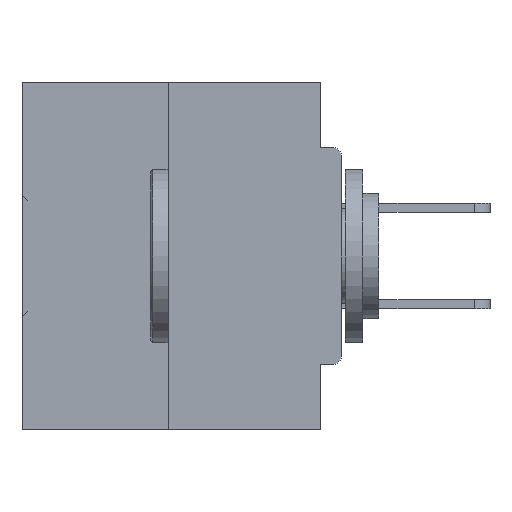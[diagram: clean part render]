
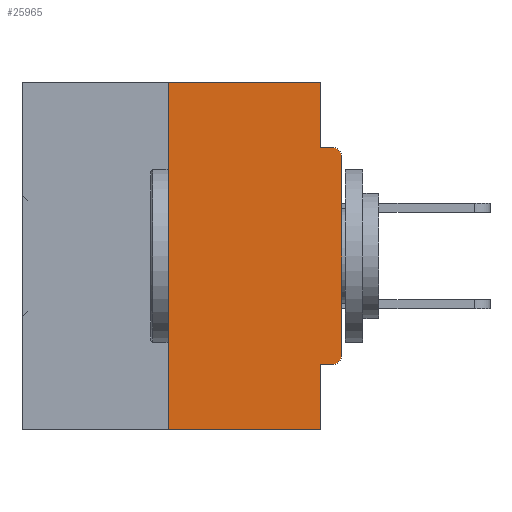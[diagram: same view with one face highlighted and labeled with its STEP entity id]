
A CAD part, left-side view. The second image highlights one B-rep face of the part: STEP entity #25965.
In plain terms, the highlighted planar face has unit normal (-1, 0, 0).
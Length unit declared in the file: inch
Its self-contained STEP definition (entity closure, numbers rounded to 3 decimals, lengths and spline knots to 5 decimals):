
#88 = VERTEX_POINT ( 'NONE', #2777 ) ;
#303 = EDGE_CURVE ( 'NONE', #88, #38447, #35368, .T. ) ;
#573 = CARTESIAN_POINT ( 'NONE',  ( 0., 0.015, -0.1085 ) ) ;
#939 = VERTEX_POINT ( 'NONE', #4171 ) ;
#961 = CARTESIAN_POINT ( 'NONE',  ( 0., 0., 0. ) ) ;
#1025 = VECTOR ( 'NONE', #41453, 39.37008 ) ;
#1994 = LINE ( 'NONE', #46334, #4847 ) ;
#2709 = ORIENTED_EDGE ( 'NONE', *, *, #18838, .T. ) ;
#2777 = CARTESIAN_POINT ( 'NONE',  ( 0., 0.015, -0.4065 ) ) ;
#3264 = LINE ( 'NONE', #10481, #41026 ) ;
#3377 = CARTESIAN_POINT ( 'NONE',  ( 0., 0.031, 0. ) ) ;
#3572 = CARTESIAN_POINT ( 'NONE',  ( 0., 0.031, -0.0935 ) ) ;
#4171 = CARTESIAN_POINT ( 'NONE',  ( 0., 0.031, 0. ) ) ;
#4847 = VECTOR ( 'NONE', #24423, 39.37008 ) ;
#6407 = ORIENTED_EDGE ( 'NONE', *, *, #303, .T. ) ;
#7286 = CARTESIAN_POINT ( 'NONE',  ( 0., 0., -0.0935 ) ) ;
#7782 = CARTESIAN_POINT ( 'NONE',  ( 0., 0.46, 0. ) ) ;
#8042 = DIRECTION ( 'NONE',  ( 0., 0., 1. ) ) ;
#8461 = CARTESIAN_POINT ( 'NONE',  ( 0., 0.031, -0.4065 ) ) ;
#8594 = VECTOR ( 'NONE', #8042, 39.37008 ) ;
#8871 = VECTOR ( 'NONE', #10265, 39.37008 ) ;
#9704 = DIRECTION ( 'NONE',  ( 0., -1., 0. ) ) ;
#10016 = AXIS2_PLACEMENT_3D ( 'NONE', #37822, #11801, #41209 ) ;
#10265 = DIRECTION ( 'NONE',  ( 0., 0., -1. ) ) ;
#10481 = CARTESIAN_POINT ( 'NONE',  ( 0., 0.031, -0.5 ) ) ;
#10542 = CARTESIAN_POINT ( 'NONE',  ( 0., 0., -0.1085 ) ) ;
#11445 = DIRECTION ( 'NONE',  ( 0., -1., 0. ) ) ;
#11801 = DIRECTION ( 'NONE',  ( 1., 0., 0. ) ) ;
#12093 = AXIS2_PLACEMENT_3D ( 'NONE', #573, #18956, #22210 ) ;
#12139 = CARTESIAN_POINT ( 'NONE',  ( 0., 0.25, 0. ) ) ;
#13243 = ORIENTED_EDGE ( 'NONE', *, *, #16351, .T. ) ;
#13870 = CARTESIAN_POINT ( 'NONE',  ( 0., 0.46, -0.5 ) ) ;
#14209 = LINE ( 'NONE', #7286, #1025 ) ;
#14239 = VERTEX_POINT ( 'NONE', #3572 ) ;
#15760 = ORIENTED_EDGE ( 'NONE', *, *, #34628, .F. ) ;
#15966 = VERTEX_POINT ( 'NONE', #8461 ) ;
#16351 = EDGE_CURVE ( 'NONE', #38447, #18301, #37714, .T. ) ;
#16870 = EDGE_CURVE ( 'NONE', #14239, #40685, #14209, .T. ) ;
#17230 = VECTOR ( 'NONE', #11445, 39.37008 ) ;
#18301 = VERTEX_POINT ( 'NONE', #10542 ) ;
#18449 = CARTESIAN_POINT ( 'NONE',  ( 0., 0.25, -0.5 ) ) ;
#18695 = FACE_OUTER_BOUND ( 'NONE', #36446, .T. ) ;
#18838 = EDGE_CURVE ( 'NONE', #18301, #40685, #26674, .T. ) ;
#18956 = DIRECTION ( 'NONE',  ( -1., 0., 0. ) ) ;
#19839 = EDGE_CURVE ( 'NONE', #88, #15966, #1994, .T. ) ;
#21056 = CARTESIAN_POINT ( 'NONE',  ( 0., 0., -0.3915 ) ) ;
#21159 = VECTOR ( 'NONE', #33905, 39.37008 ) ;
#22210 = DIRECTION ( 'NONE',  ( 0., 0., -1. ) ) ;
#22990 = EDGE_CURVE ( 'NONE', #35570, #28768, #33197, .T. ) ;
#23413 = ORIENTED_EDGE ( 'NONE', *, *, #46625, .F. ) ;
#24423 = DIRECTION ( 'NONE',  ( 0., 1., 0. ) ) ;
#25965 = ADVANCED_FACE ( 'NONE', ( #18695 ), #30326, .F. ) ;
#26558 = ORIENTED_EDGE ( 'NONE', *, *, #19839, .F. ) ;
#26566 = CARTESIAN_POINT ( 'NONE',  ( 0., 0.25, 0. ) ) ;
#26674 = CIRCLE ( 'NONE', #12093, 0.015 ) ;
#27785 = LINE ( 'NONE', #3377, #8871 ) ;
#28768 = VERTEX_POINT ( 'NONE', #12139 ) ;
#29153 = CARTESIAN_POINT ( 'NONE',  ( 0., 0.015, -0.0935 ) ) ;
#29648 = EDGE_CURVE ( 'NONE', #35570, #39472, #45876, .T. ) ;
#30326 = PLANE ( 'NONE',  #10016 ) ;
#30826 = DIRECTION ( 'NONE',  ( 0., 0., -1. ) ) ;
#31485 = CARTESIAN_POINT ( 'NONE',  ( 0., 0.015, -0.3915 ) ) ;
#31565 = LINE ( 'NONE', #7782, #17230 ) ;
#32122 = VECTOR ( 'NONE', #9704, 39.37008 ) ;
#32332 = ORIENTED_EDGE ( 'NONE', *, *, #32598, .F. ) ;
#32598 = EDGE_CURVE ( 'NONE', #28768, #939, #31565, .T. ) ;
#33197 = LINE ( 'NONE', #26566, #8594 ) ;
#33905 = DIRECTION ( 'NONE',  ( 0., 0., 1. ) ) ;
#33939 = AXIS2_PLACEMENT_3D ( 'NONE', #31485, #45355, #30826 ) ;
#34628 = EDGE_CURVE ( 'NONE', #15966, #39472, #3264, .T. ) ;
#35368 = CIRCLE ( 'NONE', #33939, 0.015 ) ;
#35570 = VERTEX_POINT ( 'NONE', #18449 ) ;
#36446 = EDGE_LOOP ( 'NONE', ( #32332, #46409, #46810, #15760, #26558, #6407, #13243, #2709, #46558, #23413 ) ) ;
#37714 = LINE ( 'NONE', #961, #21159 ) ;
#37822 = CARTESIAN_POINT ( 'NONE',  ( 0., 0.46, 0. ) ) ;
#38447 = VERTEX_POINT ( 'NONE', #21056 ) ;
#39472 = VERTEX_POINT ( 'NONE', #41717 ) ;
#39909 = DIRECTION ( 'NONE',  ( 0., 0., -1. ) ) ;
#40685 = VERTEX_POINT ( 'NONE', #29153 ) ;
#41026 = VECTOR ( 'NONE', #39909, 39.37008 ) ;
#41209 = DIRECTION ( 'NONE',  ( 0., 0., -1. ) ) ;
#41453 = DIRECTION ( 'NONE',  ( 0., -1., 0. ) ) ;
#41717 = CARTESIAN_POINT ( 'NONE',  ( 0., 0.031, -0.5 ) ) ;
#45355 = DIRECTION ( 'NONE',  ( -1., 0., 0. ) ) ;
#45876 = LINE ( 'NONE', #13870, #32122 ) ;
#46334 = CARTESIAN_POINT ( 'NONE',  ( 0., 0., -0.4065 ) ) ;
#46409 = ORIENTED_EDGE ( 'NONE', *, *, #22990, .F. ) ;
#46558 = ORIENTED_EDGE ( 'NONE', *, *, #16870, .F. ) ;
#46625 = EDGE_CURVE ( 'NONE', #939, #14239, #27785, .T. ) ;
#46810 = ORIENTED_EDGE ( 'NONE', *, *, #29648, .T. ) ;
